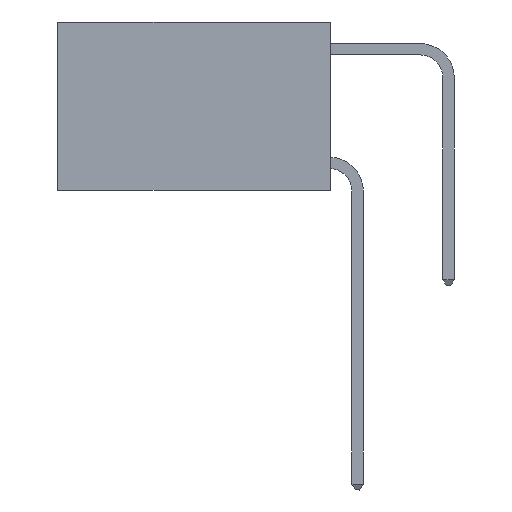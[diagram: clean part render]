
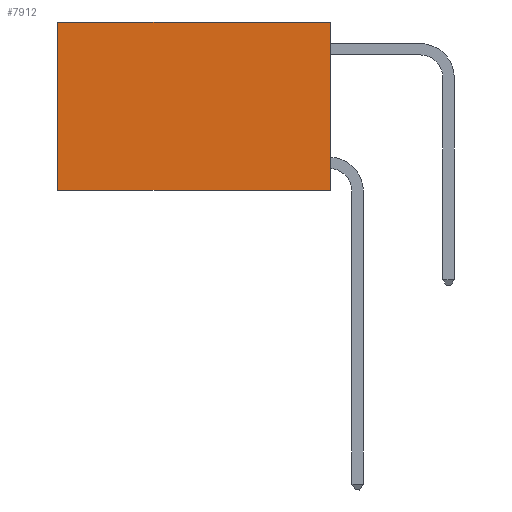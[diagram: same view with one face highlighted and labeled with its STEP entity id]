
A CAD part, left-side view. The second image highlights one B-rep face of the part: STEP entity #7912.
In plain terms, the highlighted planar face has unit normal (-1, 0, 0).
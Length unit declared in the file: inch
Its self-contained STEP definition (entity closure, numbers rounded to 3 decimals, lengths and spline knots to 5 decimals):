
#401 = ORIENTED_EDGE ( 'NONE', *, *, #15649, .F. ) ;
#454 = EDGE_LOOP ( 'NONE', ( #2314, #8330, #401, #10906 ) ) ;
#547 = DIRECTION ( 'NONE',  ( 1., 0., 0. ) ) ;
#1888 = VECTOR ( 'NONE', #2743, 39.37008 ) ;
#2041 = EDGE_CURVE ( 'NONE', #8329, #9094, #14047, .T. ) ;
#2314 = ORIENTED_EDGE ( 'NONE', *, *, #3820, .T. ) ;
#2743 = DIRECTION ( 'NONE',  ( 0., 1., 0. ) ) ;
#2963 = CARTESIAN_POINT ( 'NONE',  ( 0.2625, 0., 0. ) ) ;
#3523 = DIRECTION ( 'NONE',  ( 0., 1., 0. ) ) ;
#3820 = EDGE_CURVE ( 'NONE', #9094, #18675, #8315, .T. ) ;
#4249 = VECTOR ( 'NONE', #17006, 39.37008 ) ;
#6151 = LINE ( 'NONE', #11173, #13322 ) ;
#7912 = ADVANCED_FACE ( 'NONE', ( #12014 ), #9720, .F. ) ;
#7932 = CARTESIAN_POINT ( 'NONE',  ( 0.2625, 0., 0. ) ) ;
#7954 = AXIS2_PLACEMENT_3D ( 'NONE', #15715, #547, #11274 ) ;
#8315 = LINE ( 'NONE', #16946, #4249 ) ;
#8329 = VERTEX_POINT ( 'NONE', #13610 ) ;
#8330 = ORIENTED_EDGE ( 'NONE', *, *, #12243, .F. ) ;
#9094 = VERTEX_POINT ( 'NONE', #13828 ) ;
#9720 = PLANE ( 'NONE',  #7954 ) ;
#10906 = ORIENTED_EDGE ( 'NONE', *, *, #2041, .T. ) ;
#11173 = CARTESIAN_POINT ( 'NONE',  ( 0.2625, 0., -0.37 ) ) ;
#11274 = DIRECTION ( 'NONE',  ( 0., 0., -1. ) ) ;
#11644 = CARTESIAN_POINT ( 'NONE',  ( 0.2625, 0., -0.37 ) ) ;
#12009 = VECTOR ( 'NONE', #16970, 39.37008 ) ;
#12014 = FACE_OUTER_BOUND ( 'NONE', #454, .T. ) ;
#12243 = EDGE_CURVE ( 'NONE', #16578, #18675, #6151, .T. ) ;
#12932 = LINE ( 'NONE', #7932, #12009 ) ;
#13322 = VECTOR ( 'NONE', #3523, 39.37008 ) ;
#13610 = CARTESIAN_POINT ( 'NONE',  ( 0.2625, 0., 0. ) ) ;
#13828 = CARTESIAN_POINT ( 'NONE',  ( 0.2625, 0.6, 0. ) ) ;
#14047 = LINE ( 'NONE', #2963, #1888 ) ;
#15012 = CARTESIAN_POINT ( 'NONE',  ( 0.2625, 0.6, -0.37 ) ) ;
#15649 = EDGE_CURVE ( 'NONE', #8329, #16578, #12932, .T. ) ;
#15715 = CARTESIAN_POINT ( 'NONE',  ( 0.2625, 0., 0. ) ) ;
#16578 = VERTEX_POINT ( 'NONE', #11644 ) ;
#16946 = CARTESIAN_POINT ( 'NONE',  ( 0.2625, 0.6, 0. ) ) ;
#16970 = DIRECTION ( 'NONE',  ( 0., 0., -1. ) ) ;
#17006 = DIRECTION ( 'NONE',  ( 0., 0., -1. ) ) ;
#18675 = VERTEX_POINT ( 'NONE', #15012 ) ;
